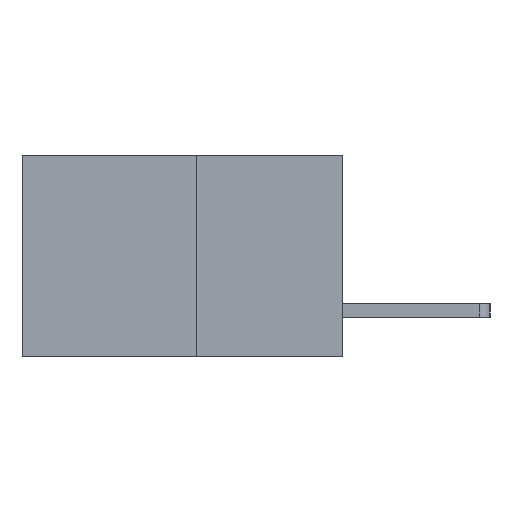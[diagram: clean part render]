
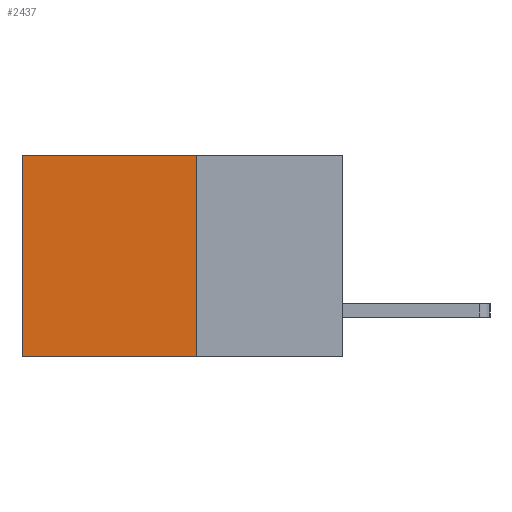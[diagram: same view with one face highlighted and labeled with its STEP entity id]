
A CAD part, left-side view. The second image highlights one B-rep face of the part: STEP entity #2437.
In plain terms, the highlighted planar face has unit normal (-1, 0, 0).
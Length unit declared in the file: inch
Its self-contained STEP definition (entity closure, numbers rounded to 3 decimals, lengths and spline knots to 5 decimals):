
#1207 = CARTESIAN_POINT ( 'NONE',  ( 0.277, 0.59, -0.37 ) ) ;
#1381 = LINE ( 'NONE', #8127, #5503 ) ;
#1509 = VERTEX_POINT ( 'NONE', #6550 ) ;
#2020 = LINE ( 'NONE', #2907, #7861 ) ;
#2088 = DIRECTION ( 'NONE',  ( 0., 0., -1. ) ) ;
#2331 = CARTESIAN_POINT ( 'NONE',  ( 0.277, 0.27, -0.37 ) ) ;
#2372 = EDGE_LOOP ( 'NONE', ( #8765, #8771, #9750, #9644 ) ) ;
#2437 = ADVANCED_FACE ( 'NONE', ( #8822 ), #4117, .F. ) ;
#2907 = CARTESIAN_POINT ( 'NONE',  ( 0.277, 0.27, 0. ) ) ;
#3208 = DIRECTION ( 'NONE',  ( 0., 1., 0. ) ) ;
#3438 = EDGE_CURVE ( 'NONE', #1509, #5676, #1381, .T. ) ;
#3873 = DIRECTION ( 'NONE',  ( 0., 0., -1. ) ) ;
#3906 = VERTEX_POINT ( 'NONE', #5759 ) ;
#4117 = PLANE ( 'NONE',  #7775 ) ;
#5144 = EDGE_CURVE ( 'NONE', #9925, #3906, #8384, .T. ) ;
#5207 = DIRECTION ( 'NONE',  ( 0., 1., 0. ) ) ;
#5503 = VECTOR ( 'NONE', #3873, 39.37008 ) ;
#5676 = VERTEX_POINT ( 'NONE', #1207 ) ;
#5759 = CARTESIAN_POINT ( 'NONE',  ( 0.277, 0.27, -0.37 ) ) ;
#5841 = CARTESIAN_POINT ( 'NONE',  ( 0.277, 0.27, -0.37 ) ) ;
#6175 = VECTOR ( 'NONE', #2088, 39.37008 ) ;
#6382 = EDGE_CURVE ( 'NONE', #3906, #5676, #7114, .T. ) ;
#6550 = CARTESIAN_POINT ( 'NONE',  ( 0.277, 0.59, 0. ) ) ;
#7114 = LINE ( 'NONE', #2331, #9125 ) ;
#7775 = AXIS2_PLACEMENT_3D ( 'NONE', #8627, #9198, #8332 ) ;
#7861 = VECTOR ( 'NONE', #5207, 39.37008 ) ;
#8127 = CARTESIAN_POINT ( 'NONE',  ( 0.277, 0.59, -0.37 ) ) ;
#8332 = DIRECTION ( 'NONE',  ( 0., 0., -1. ) ) ;
#8384 = LINE ( 'NONE', #5841, #6175 ) ;
#8449 = CARTESIAN_POINT ( 'NONE',  ( 0.277, 0.27, 0. ) ) ;
#8627 = CARTESIAN_POINT ( 'NONE',  ( 0.277, 0.27, -0.37 ) ) ;
#8765 = ORIENTED_EDGE ( 'NONE', *, *, #3438, .T. ) ;
#8771 = ORIENTED_EDGE ( 'NONE', *, *, #6382, .F. ) ;
#8822 = FACE_OUTER_BOUND ( 'NONE', #2372, .T. ) ;
#9125 = VECTOR ( 'NONE', #3208, 39.37008 ) ;
#9198 = DIRECTION ( 'NONE',  ( 1., 0., 0. ) ) ;
#9644 = ORIENTED_EDGE ( 'NONE', *, *, #9673, .T. ) ;
#9673 = EDGE_CURVE ( 'NONE', #9925, #1509, #2020, .T. ) ;
#9750 = ORIENTED_EDGE ( 'NONE', *, *, #5144, .F. ) ;
#9925 = VERTEX_POINT ( 'NONE', #8449 ) ;
